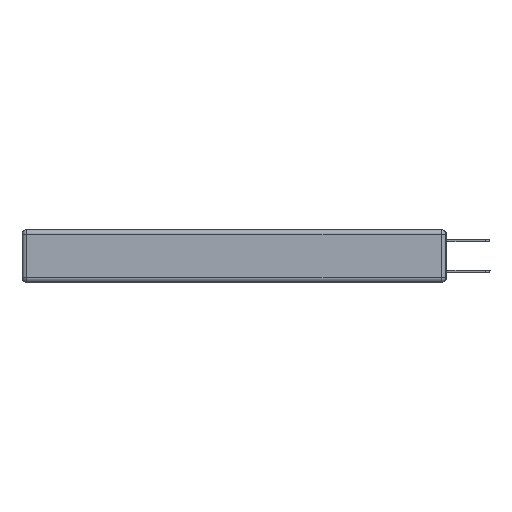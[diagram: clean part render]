
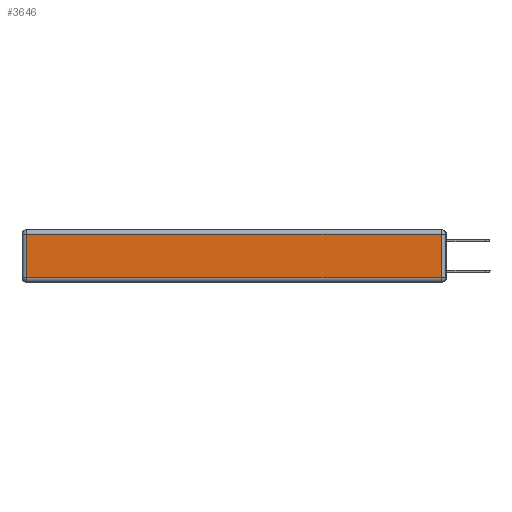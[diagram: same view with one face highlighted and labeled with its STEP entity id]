
A CAD part, left-side view. The second image highlights one B-rep face of the part: STEP entity #3646.
In plain terms, the highlighted planar face has unit normal (-1, 0, 0).
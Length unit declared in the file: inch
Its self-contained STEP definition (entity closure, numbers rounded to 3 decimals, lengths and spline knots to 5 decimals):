
#872 = CARTESIAN_POINT ( 'NONE',  ( 0., 2.72, -0.343 ) ) ;
#1006 = FACE_OUTER_BOUND ( 'NONE', #8862, .T. ) ;
#1727 = ORIENTED_EDGE ( 'NONE', *, *, #22622, .T. ) ;
#2181 = PLANE ( 'NONE',  #8288 ) ;
#2736 = DIRECTION ( 'NONE',  ( 0., 0., -1. ) ) ;
#3646 = ADVANCED_FACE ( 'NONE', ( #1006 ), #2181, .T. ) ;
#3805 = VECTOR ( 'NONE', #10215, 39.37008 ) ;
#4916 = ORIENTED_EDGE ( 'NONE', *, *, #20476, .T. ) ;
#5514 = ORIENTED_EDGE ( 'NONE', *, *, #17824, .T. ) ;
#5980 = DIRECTION ( 'NONE',  ( -1., 0., 0. ) ) ;
#7085 = CARTESIAN_POINT ( 'NONE',  ( 0., 0.03, -0.03 ) ) ;
#7460 = CARTESIAN_POINT ( 'NONE',  ( 0., 2.72, -0.03 ) ) ;
#7478 = VECTOR ( 'NONE', #16666, 39.37008 ) ;
#8288 = AXIS2_PLACEMENT_3D ( 'NONE', #17105, #5980, #11572 ) ;
#8862 = EDGE_LOOP ( 'NONE', ( #22428, #4916, #1727, #5514 ) ) ;
#9481 = LINE ( 'NONE', #18380, #7478 ) ;
#10024 = VERTEX_POINT ( 'NONE', #10443 ) ;
#10200 = CARTESIAN_POINT ( 'NONE',  ( 0., 2.72, -0.313 ) ) ;
#10215 = DIRECTION ( 'NONE',  ( 0., 0., 1. ) ) ;
#10443 = CARTESIAN_POINT ( 'NONE',  ( 0., 0.03, -0.313 ) ) ;
#11572 = DIRECTION ( 'NONE',  ( 0., 0., 1. ) ) ;
#13033 = EDGE_CURVE ( 'NONE', #18993, #10024, #18790, .T. ) ;
#13126 = VERTEX_POINT ( 'NONE', #7460 ) ;
#13661 = LINE ( 'NONE', #16506, #3805 ) ;
#15001 = DIRECTION ( 'NONE',  ( 0., -1., 0. ) ) ;
#16375 = VERTEX_POINT ( 'NONE', #7085 ) ;
#16506 = CARTESIAN_POINT ( 'NONE',  ( 0., 0.03, -0.343 ) ) ;
#16666 = DIRECTION ( 'NONE',  ( 0., 1., 0. ) ) ;
#17105 = CARTESIAN_POINT ( 'NONE',  ( 0., 0., -0.343 ) ) ;
#17824 = EDGE_CURVE ( 'NONE', #13126, #18993, #23689, .T. ) ;
#18380 = CARTESIAN_POINT ( 'NONE',  ( 0., 2.75, -0.03 ) ) ;
#18790 = LINE ( 'NONE', #20539, #22241 ) ;
#18993 = VERTEX_POINT ( 'NONE', #10200 ) ;
#19370 = VECTOR ( 'NONE', #2736, 39.37008 ) ;
#20476 = EDGE_CURVE ( 'NONE', #10024, #16375, #13661, .T. ) ;
#20539 = CARTESIAN_POINT ( 'NONE',  ( 0., 0., -0.313 ) ) ;
#22241 = VECTOR ( 'NONE', #15001, 39.37008 ) ;
#22428 = ORIENTED_EDGE ( 'NONE', *, *, #13033, .T. ) ;
#22622 = EDGE_CURVE ( 'NONE', #16375, #13126, #9481, .T. ) ;
#23689 = LINE ( 'NONE', #872, #19370 ) ;
